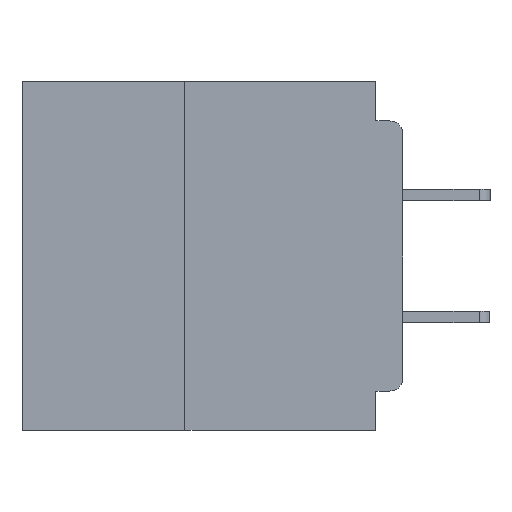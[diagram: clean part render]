
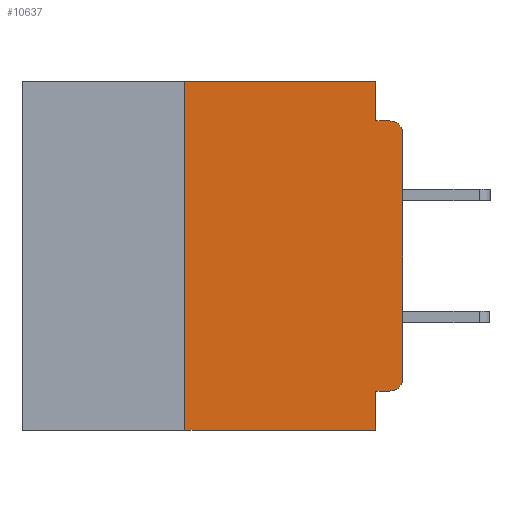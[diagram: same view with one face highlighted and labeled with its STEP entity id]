
A CAD part, left-side view. The second image highlights one B-rep face of the part: STEP entity #10637.
In plain terms, the highlighted planar face has unit normal (-1, 0, 0).
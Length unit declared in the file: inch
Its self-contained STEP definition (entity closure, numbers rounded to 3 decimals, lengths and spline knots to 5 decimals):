
#1217 = VERTEX_POINT ( 'NONE', #13294 ) ;
#1266 = ORIENTED_EDGE ( 'NONE', *, *, #7587, .F. ) ;
#1489 = DIRECTION ( 'NONE',  ( 0., 0., 1. ) ) ;
#1559 = AXIS2_PLACEMENT_3D ( 'NONE', #12978, #35878, #16295 ) ;
#1640 = VERTEX_POINT ( 'NONE', #31641 ) ;
#1700 = EDGE_LOOP ( 'NONE', ( #11613, #3839, #39808, #32110, #34176, #1266, #28546, #3336, #31618, #23982 ) ) ;
#2162 = DIRECTION ( 'NONE',  ( -1., 0., 0. ) ) ;
#3216 = VECTOR ( 'NONE', #35101, 39.37008 ) ;
#3336 = ORIENTED_EDGE ( 'NONE', *, *, #29663, .F. ) ;
#3399 = VERTEX_POINT ( 'NONE', #42530 ) ;
#3623 = LINE ( 'NONE', #9159, #27792 ) ;
#3645 = VECTOR ( 'NONE', #31697, 39.37008 ) ;
#3839 = ORIENTED_EDGE ( 'NONE', *, *, #20713, .T. ) ;
#6445 = LINE ( 'NONE', #35096, #31610 ) ;
#6574 = LINE ( 'NONE', #21226, #40003 ) ;
#7587 = EDGE_CURVE ( 'NONE', #1640, #3399, #32428, .T. ) ;
#8184 = VERTEX_POINT ( 'NONE', #29761 ) ;
#8872 = VECTOR ( 'NONE', #14461, 39.37008 ) ;
#9159 = CARTESIAN_POINT ( 'NONE',  ( 0., 0.437, 0. ) ) ;
#9552 = EDGE_CURVE ( 'NONE', #31668, #8184, #6574, .T. ) ;
#10194 = CARTESIAN_POINT ( 'NONE',  ( 0., 0.437, 0. ) ) ;
#10637 = ADVANCED_FACE ( 'NONE', ( #20738 ), #29822, .F. ) ;
#11267 = CARTESIAN_POINT ( 'NONE',  ( 0., 0., -0.34 ) ) ;
#11613 = ORIENTED_EDGE ( 'NONE', *, *, #9552, .T. ) ;
#11991 = VERTEX_POINT ( 'NONE', #23581 ) ;
#12474 = DIRECTION ( 'NONE',  ( 0., -1., 0. ) ) ;
#12978 = CARTESIAN_POINT ( 'NONE',  ( 0., 0.015, -0.06 ) ) ;
#13294 = CARTESIAN_POINT ( 'NONE',  ( 0., 0.031, 0. ) ) ;
#13464 = CARTESIAN_POINT ( 'NONE',  ( 0., 0.031, -0.4 ) ) ;
#13501 = DIRECTION ( 'NONE',  ( 1., 0., 0. ) ) ;
#13985 = VECTOR ( 'NONE', #36381, 39.37008 ) ;
#14342 = CARTESIAN_POINT ( 'NONE',  ( 0., 0.015, -0.045 ) ) ;
#14461 = DIRECTION ( 'NONE',  ( 0., -1., 0. ) ) ;
#16248 = AXIS2_PLACEMENT_3D ( 'NONE', #10194, #13501, #36383 ) ;
#16295 = DIRECTION ( 'NONE',  ( 0., 0., -1. ) ) ;
#16932 = CARTESIAN_POINT ( 'NONE',  ( 0., 0.25, -0.4 ) ) ;
#17581 = LINE ( 'NONE', #20893, #8872 ) ;
#18649 = CARTESIAN_POINT ( 'NONE',  ( 0., 0.031, -0.4 ) ) ;
#19800 = VERTEX_POINT ( 'NONE', #14342 ) ;
#20713 = EDGE_CURVE ( 'NONE', #8184, #19800, #25125, .T. ) ;
#20738 = FACE_OUTER_BOUND ( 'NONE', #1700, .T. ) ;
#20893 = CARTESIAN_POINT ( 'NONE',  ( 0., 0.437, -0.4 ) ) ;
#21226 = CARTESIAN_POINT ( 'NONE',  ( 0., 0., 0. ) ) ;
#21388 = AXIS2_PLACEMENT_3D ( 'NONE', #21878, #2162, #25200 ) ;
#21878 = CARTESIAN_POINT ( 'NONE',  ( 0., 0.015, -0.34 ) ) ;
#23581 = CARTESIAN_POINT ( 'NONE',  ( 0., 0.031, -0.355 ) ) ;
#23622 = EDGE_CURVE ( 'NONE', #1640, #28102, #17581, .T. ) ;
#23982 = ORIENTED_EDGE ( 'NONE', *, *, #36879, .T. ) ;
#24422 = CARTESIAN_POINT ( 'NONE',  ( 0., 0., -0.045 ) ) ;
#25081 = LINE ( 'NONE', #24422, #32735 ) ;
#25125 = CIRCLE ( 'NONE', #1559, 0.015 ) ;
#25200 = DIRECTION ( 'NONE',  ( 0., 0., -1. ) ) ;
#27661 = DIRECTION ( 'NONE',  ( 0., -1., 0. ) ) ;
#27792 = VECTOR ( 'NONE', #12474, 39.37008 ) ;
#27872 = EDGE_CURVE ( 'NONE', #31320, #11991, #6445, .T. ) ;
#28102 = VERTEX_POINT ( 'NONE', #13464 ) ;
#28546 = ORIENTED_EDGE ( 'NONE', *, *, #23622, .T. ) ;
#28851 = LINE ( 'NONE', #41600, #3645 ) ;
#29663 = EDGE_CURVE ( 'NONE', #11991, #28102, #38140, .T. ) ;
#29761 = CARTESIAN_POINT ( 'NONE',  ( 0., 0., -0.06 ) ) ;
#29822 = PLANE ( 'NONE',  #16248 ) ;
#31320 = VERTEX_POINT ( 'NONE', #42251 ) ;
#31610 = VECTOR ( 'NONE', #38379, 39.37008 ) ;
#31618 = ORIENTED_EDGE ( 'NONE', *, *, #27872, .F. ) ;
#31641 = CARTESIAN_POINT ( 'NONE',  ( 0., 0.25, -0.4 ) ) ;
#31668 = VERTEX_POINT ( 'NONE', #11267 ) ;
#31697 = DIRECTION ( 'NONE',  ( 0., 0., -1. ) ) ;
#32110 = ORIENTED_EDGE ( 'NONE', *, *, #40556, .F. ) ;
#32428 = LINE ( 'NONE', #16932, #13985 ) ;
#32545 = CIRCLE ( 'NONE', #21388, 0.015 ) ;
#32713 = VERTEX_POINT ( 'NONE', #40138 ) ;
#32735 = VECTOR ( 'NONE', #27661, 39.37008 ) ;
#32814 = EDGE_CURVE ( 'NONE', #32713, #19800, #25081, .T. ) ;
#34176 = ORIENTED_EDGE ( 'NONE', *, *, #39251, .F. ) ;
#35096 = CARTESIAN_POINT ( 'NONE',  ( 0., 0., -0.355 ) ) ;
#35101 = DIRECTION ( 'NONE',  ( 0., 0., -1. ) ) ;
#35878 = DIRECTION ( 'NONE',  ( -1., 0., 0. ) ) ;
#36381 = DIRECTION ( 'NONE',  ( 0., 0., 1. ) ) ;
#36383 = DIRECTION ( 'NONE',  ( 0., 0., -1. ) ) ;
#36879 = EDGE_CURVE ( 'NONE', #31320, #31668, #32545, .T. ) ;
#38140 = LINE ( 'NONE', #18649, #3216 ) ;
#38379 = DIRECTION ( 'NONE',  ( 0., 1., 0. ) ) ;
#39251 = EDGE_CURVE ( 'NONE', #3399, #1217, #3623, .T. ) ;
#39808 = ORIENTED_EDGE ( 'NONE', *, *, #32814, .F. ) ;
#40003 = VECTOR ( 'NONE', #1489, 39.37008 ) ;
#40138 = CARTESIAN_POINT ( 'NONE',  ( 0., 0.031, -0.045 ) ) ;
#40556 = EDGE_CURVE ( 'NONE', #1217, #32713, #28851, .T. ) ;
#41600 = CARTESIAN_POINT ( 'NONE',  ( 0., 0.031, 0. ) ) ;
#42251 = CARTESIAN_POINT ( 'NONE',  ( 0., 0.015, -0.355 ) ) ;
#42530 = CARTESIAN_POINT ( 'NONE',  ( 0., 0.25, 0. ) ) ;
